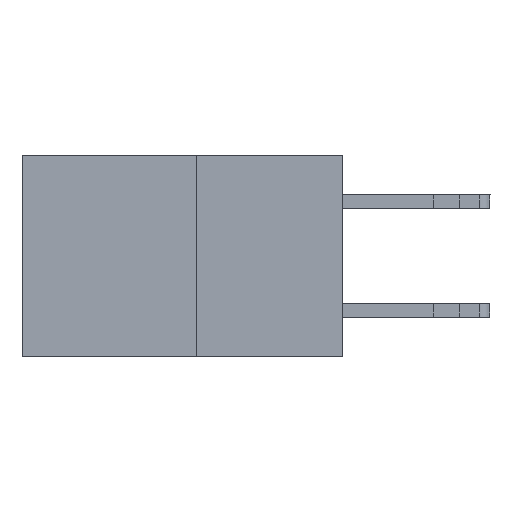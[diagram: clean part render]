
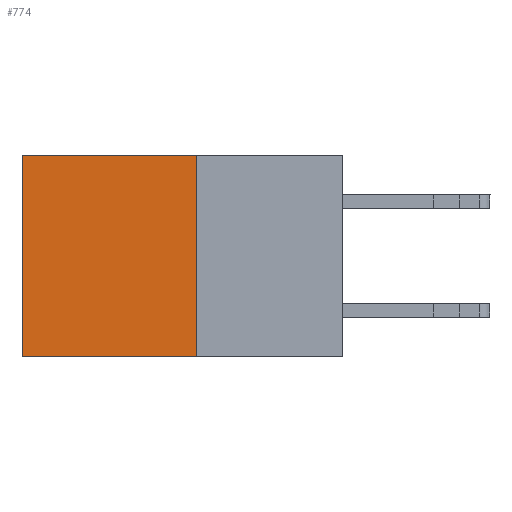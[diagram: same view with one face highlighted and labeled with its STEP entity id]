
A CAD part, left-side view. The second image highlights one B-rep face of the part: STEP entity #774.
In plain terms, the highlighted planar face has unit normal (-1, 0, 0).
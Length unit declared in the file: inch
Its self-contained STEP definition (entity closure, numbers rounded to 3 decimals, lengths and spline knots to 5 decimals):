
#774 = ADVANCED_FACE ( 'NONE', ( #15803 ), #2538, .F. ) ;
#1362 = LINE ( 'NONE', #11591, #14651 ) ;
#2538 = PLANE ( 'NONE',  #15619 ) ;
#4232 = VERTEX_POINT ( 'NONE', #25099 ) ;
#6385 = ORIENTED_EDGE ( 'NONE', *, *, #31903, .F. ) ;
#6434 = CARTESIAN_POINT ( 'NONE',  ( 0.277, 0.27, -0.37 ) ) ;
#7733 = CARTESIAN_POINT ( 'NONE',  ( 0.277, 0.27, -0.37 ) ) ;
#9245 = VECTOR ( 'NONE', #13395, 39.37008 ) ;
#9730 = EDGE_CURVE ( 'NONE', #16807, #29720, #27172, .T. ) ;
#11074 = ORIENTED_EDGE ( 'NONE', *, *, #15159, .T. ) ;
#11591 = CARTESIAN_POINT ( 'NONE',  ( 0.277, 0.27, -0.37 ) ) ;
#12238 = CARTESIAN_POINT ( 'NONE',  ( 0.277, 0.27, -0.37 ) ) ;
#13064 = CARTESIAN_POINT ( 'NONE',  ( 0.277, 0.59, -0.37 ) ) ;
#13395 = DIRECTION ( 'NONE',  ( 0., 0., -1. ) ) ;
#14249 = VECTOR ( 'NONE', #28098, 39.37008 ) ;
#14651 = VECTOR ( 'NONE', #31591, 39.37008 ) ;
#15159 = EDGE_CURVE ( 'NONE', #16807, #4232, #15517, .T. ) ;
#15517 = LINE ( 'NONE', #18032, #14249 ) ;
#15619 = AXIS2_PLACEMENT_3D ( 'NONE', #7733, #17981, #28201 ) ;
#15803 = FACE_OUTER_BOUND ( 'NONE', #30977, .T. ) ;
#16807 = VERTEX_POINT ( 'NONE', #19042 ) ;
#17981 = DIRECTION ( 'NONE',  ( 1., 0., 0. ) ) ;
#18032 = CARTESIAN_POINT ( 'NONE',  ( 0.277, 0.27, 0. ) ) ;
#19042 = CARTESIAN_POINT ( 'NONE',  ( 0.277, 0.27, 0. ) ) ;
#21061 = ORIENTED_EDGE ( 'NONE', *, *, #9730, .F. ) ;
#21693 = VERTEX_POINT ( 'NONE', #13064 ) ;
#22485 = DIRECTION ( 'NONE',  ( 0., 0., -1. ) ) ;
#25099 = CARTESIAN_POINT ( 'NONE',  ( 0.277, 0.59, 0. ) ) ;
#25391 = VECTOR ( 'NONE', #22485, 39.37008 ) ;
#26138 = EDGE_CURVE ( 'NONE', #4232, #21693, #29167, .T. ) ;
#26634 = CARTESIAN_POINT ( 'NONE',  ( 0.277, 0.59, -0.37 ) ) ;
#27172 = LINE ( 'NONE', #12238, #25391 ) ;
#27572 = ORIENTED_EDGE ( 'NONE', *, *, #26138, .T. ) ;
#28098 = DIRECTION ( 'NONE',  ( 0., 1., 0. ) ) ;
#28201 = DIRECTION ( 'NONE',  ( 0., 0., -1. ) ) ;
#29167 = LINE ( 'NONE', #26634, #9245 ) ;
#29720 = VERTEX_POINT ( 'NONE', #6434 ) ;
#30977 = EDGE_LOOP ( 'NONE', ( #27572, #6385, #21061, #11074 ) ) ;
#31591 = DIRECTION ( 'NONE',  ( 0., 1., 0. ) ) ;
#31903 = EDGE_CURVE ( 'NONE', #29720, #21693, #1362, .T. ) ;
